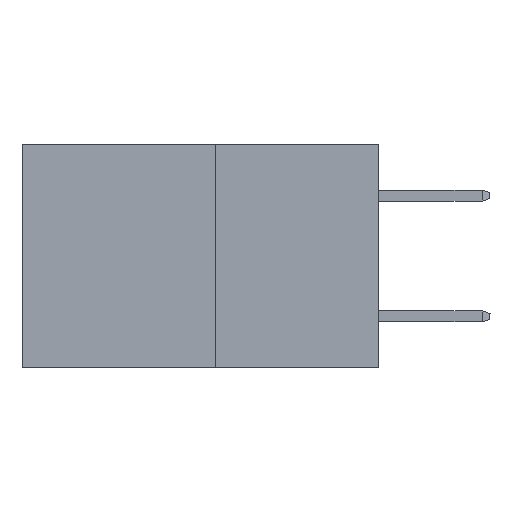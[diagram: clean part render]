
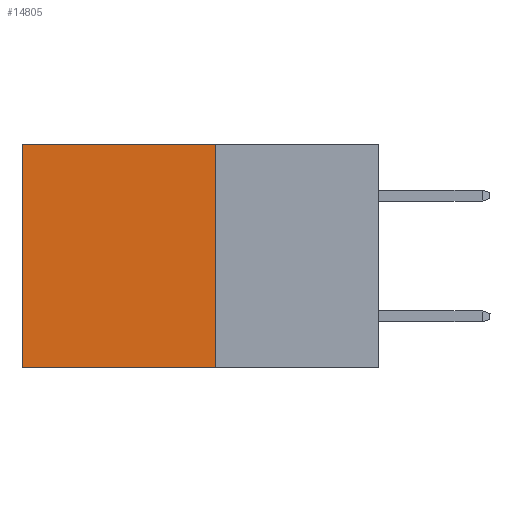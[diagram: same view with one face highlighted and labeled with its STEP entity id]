
A CAD part, left-side view. The second image highlights one B-rep face of the part: STEP entity #14805.
In plain terms, the highlighted planar face has unit normal (-1, 0, 0).
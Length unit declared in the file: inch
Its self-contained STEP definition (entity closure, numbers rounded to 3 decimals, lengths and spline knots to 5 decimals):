
#45 = CARTESIAN_POINT ( 'NONE',  ( 0.277, 0.27, -0.37 ) ) ;
#343 = EDGE_CURVE ( 'NONE', #7522, #11657, #15224, .T. ) ;
#462 = VERTEX_POINT ( 'NONE', #15144 ) ;
#984 = EDGE_LOOP ( 'NONE', ( #14613, #4810, #11708, #10011 ) ) ;
#1015 = LINE ( 'NONE', #4178, #4243 ) ;
#1386 = FACE_OUTER_BOUND ( 'NONE', #984, .T. ) ;
#1429 = VECTOR ( 'NONE', #5949, 39.37008 ) ;
#1653 = DIRECTION ( 'NONE',  ( 0., 0., -1. ) ) ;
#1721 = VECTOR ( 'NONE', #12290, 39.37008 ) ;
#2957 = CARTESIAN_POINT ( 'NONE',  ( 0.277, 0.27, -0.37 ) ) ;
#3203 = DIRECTION ( 'NONE',  ( 0., 0., -1. ) ) ;
#3391 = CARTESIAN_POINT ( 'NONE',  ( 0.277, 0.27, 0. ) ) ;
#4178 = CARTESIAN_POINT ( 'NONE',  ( 0.277, 0.27, -0.37 ) ) ;
#4243 = VECTOR ( 'NONE', #14827, 39.37008 ) ;
#4810 = ORIENTED_EDGE ( 'NONE', *, *, #12030, .F. ) ;
#5949 = DIRECTION ( 'NONE',  ( 0., 1., 0. ) ) ;
#6905 = VERTEX_POINT ( 'NONE', #11119 ) ;
#6933 = EDGE_CURVE ( 'NONE', #11657, #462, #16336, .T. ) ;
#7061 = CARTESIAN_POINT ( 'NONE',  ( 0.277, 0.27, 0. ) ) ;
#7522 = VERTEX_POINT ( 'NONE', #7061 ) ;
#8487 = PLANE ( 'NONE',  #13735 ) ;
#8889 = CARTESIAN_POINT ( 'NONE',  ( 0.277, 0.59, 0. ) ) ;
#9498 = VECTOR ( 'NONE', #3203, 39.37008 ) ;
#9821 = DIRECTION ( 'NONE',  ( 1., 0., 0. ) ) ;
#10011 = ORIENTED_EDGE ( 'NONE', *, *, #343, .T. ) ;
#11119 = CARTESIAN_POINT ( 'NONE',  ( 0.277, 0.27, -0.37 ) ) ;
#11356 = EDGE_CURVE ( 'NONE', #7522, #6905, #12909, .T. ) ;
#11657 = VERTEX_POINT ( 'NONE', #8889 ) ;
#11708 = ORIENTED_EDGE ( 'NONE', *, *, #11356, .F. ) ;
#12030 = EDGE_CURVE ( 'NONE', #6905, #462, #1015, .T. ) ;
#12290 = DIRECTION ( 'NONE',  ( 0., 0., -1. ) ) ;
#12909 = LINE ( 'NONE', #45, #1721 ) ;
#13735 = AXIS2_PLACEMENT_3D ( 'NONE', #2957, #9821, #1653 ) ;
#13797 = CARTESIAN_POINT ( 'NONE',  ( 0.277, 0.59, -0.37 ) ) ;
#14613 = ORIENTED_EDGE ( 'NONE', *, *, #6933, .T. ) ;
#14805 = ADVANCED_FACE ( 'NONE', ( #1386 ), #8487, .F. ) ;
#14827 = DIRECTION ( 'NONE',  ( 0., 1., 0. ) ) ;
#15144 = CARTESIAN_POINT ( 'NONE',  ( 0.277, 0.59, -0.37 ) ) ;
#15224 = LINE ( 'NONE', #3391, #1429 ) ;
#16336 = LINE ( 'NONE', #13797, #9498 ) ;
